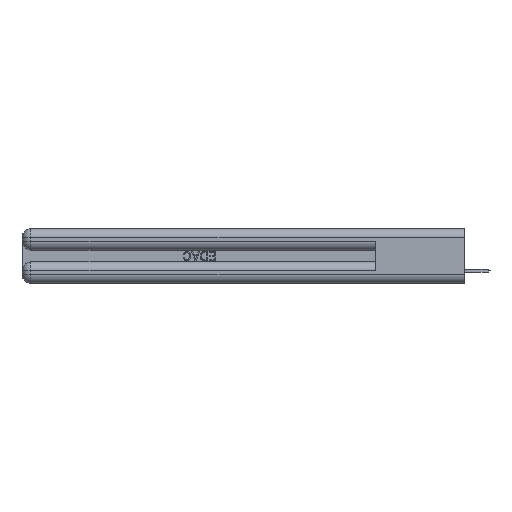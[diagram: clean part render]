
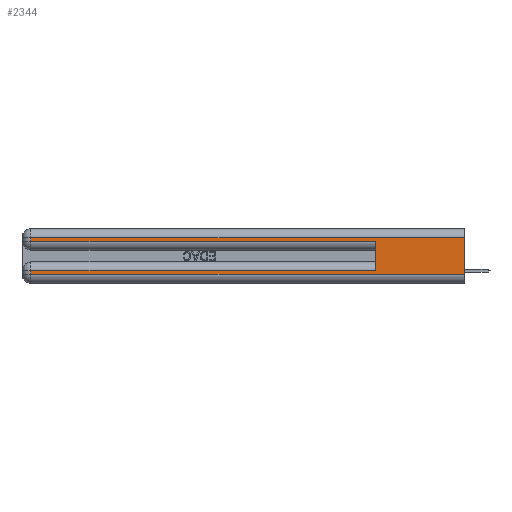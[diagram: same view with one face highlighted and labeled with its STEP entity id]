
A CAD part, left-side view. The second image highlights one B-rep face of the part: STEP entity #2344.
In plain terms, the highlighted planar face has unit normal (-1, 0, 0).
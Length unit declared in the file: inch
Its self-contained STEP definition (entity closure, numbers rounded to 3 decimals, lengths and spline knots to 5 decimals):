
#362 = VERTEX_POINT ( 'NONE', #38964 ) ;
#955 = EDGE_CURVE ( 'NONE', #15103, #29550, #20233, .T. ) ;
#1811 = CARTESIAN_POINT ( 'NONE',  ( 0., 2.94, 0.31 ) ) ;
#2344 = ADVANCED_FACE ( 'NONE', ( #28671 ), #14030, .F. ) ;
#2415 = ORIENTED_EDGE ( 'NONE', *, *, #22711, .F. ) ;
#2504 = LINE ( 'NONE', #26311, #26095 ) ;
#2969 = DIRECTION ( 'NONE',  ( 0., 0., -1. ) ) ;
#3115 = DIRECTION ( 'NONE',  ( 0., -1., 0. ) ) ;
#3134 = VERTEX_POINT ( 'NONE', #21106 ) ;
#3225 = EDGE_CURVE ( 'NONE', #16773, #38632, #2504, .T. ) ;
#3270 = DIRECTION ( 'NONE',  ( 0., 0., -1. ) ) ;
#4469 = CARTESIAN_POINT ( 'NONE',  ( 0., 2.94, 0.085 ) ) ;
#4632 = ORIENTED_EDGE ( 'NONE', *, *, #32119, .T. ) ;
#5028 = LINE ( 'NONE', #17285, #19050 ) ;
#5137 = DIRECTION ( 'NONE',  ( 0., 0., 1. ) ) ;
#5389 = DIRECTION ( 'NONE',  ( 0., 0., -1. ) ) ;
#7161 = VECTOR ( 'NONE', #3270, 39.37008 ) ;
#7966 = DIRECTION ( 'NONE',  ( 0., 1., 0. ) ) ;
#8090 = CARTESIAN_POINT ( 'NONE',  ( 0., 2.94, 0.06 ) ) ;
#8516 = DIRECTION ( 'NONE',  ( 0., 1., 0. ) ) ;
#8876 = CARTESIAN_POINT ( 'NONE',  ( 0., 0.6, 0.085 ) ) ;
#9044 = VERTEX_POINT ( 'NONE', #1811 ) ;
#10398 = EDGE_CURVE ( 'NONE', #43129, #38632, #41412, .T. ) ;
#12212 = EDGE_CURVE ( 'NONE', #29550, #43129, #5028, .T. ) ;
#14030 = PLANE ( 'NONE',  #15608 ) ;
#15103 = VERTEX_POINT ( 'NONE', #8876 ) ;
#15608 = AXIS2_PLACEMENT_3D ( 'NONE', #43233, #17788, #35631 ) ;
#16773 = VERTEX_POINT ( 'NONE', #19461 ) ;
#17285 = CARTESIAN_POINT ( 'NONE',  ( 0., 2.94, 0.37 ) ) ;
#17788 = DIRECTION ( 'NONE',  ( 1., 0., 0. ) ) ;
#19050 = VECTOR ( 'NONE', #2969, 39.37008 ) ;
#19461 = CARTESIAN_POINT ( 'NONE',  ( 0., 0., 0.31 ) ) ;
#20233 = LINE ( 'NONE', #29545, #36537 ) ;
#20673 = LINE ( 'NONE', #24368, #7161 ) ;
#21061 = CARTESIAN_POINT ( 'NONE',  ( 0., 0., 0.285 ) ) ;
#21106 = CARTESIAN_POINT ( 'NONE',  ( 0., 0.6, 0.285 ) ) ;
#21203 = VECTOR ( 'NONE', #8516, 39.37008 ) ;
#21588 = LINE ( 'NONE', #26998, #41427 ) ;
#22084 = VECTOR ( 'NONE', #33258, 39.37008 ) ;
#22711 = EDGE_CURVE ( 'NONE', #15103, #3134, #21588, .T. ) ;
#23289 = LINE ( 'NONE', #21061, #41484 ) ;
#23952 = ORIENTED_EDGE ( 'NONE', *, *, #37286, .T. ) ;
#23984 = LINE ( 'NONE', #33750, #21203 ) ;
#24368 = CARTESIAN_POINT ( 'NONE',  ( 0., 2.94, 0.37 ) ) ;
#25414 = ORIENTED_EDGE ( 'NONE', *, *, #955, .T. ) ;
#25744 = ORIENTED_EDGE ( 'NONE', *, *, #10398, .T. ) ;
#26095 = VECTOR ( 'NONE', #5389, 39.37008 ) ;
#26311 = CARTESIAN_POINT ( 'NONE',  ( 0., 0., 0.37 ) ) ;
#26807 = ORIENTED_EDGE ( 'NONE', *, *, #12212, .T. ) ;
#26998 = CARTESIAN_POINT ( 'NONE',  ( 0., 0.6, 0.145 ) ) ;
#28671 = FACE_OUTER_BOUND ( 'NONE', #34895, .T. ) ;
#29325 = CARTESIAN_POINT ( 'NONE',  ( 0., 0., 0.06 ) ) ;
#29545 = CARTESIAN_POINT ( 'NONE',  ( 0., 0., 0.085 ) ) ;
#29550 = VERTEX_POINT ( 'NONE', #4469 ) ;
#32119 = EDGE_CURVE ( 'NONE', #9044, #362, #20673, .T. ) ;
#32434 = EDGE_CURVE ( 'NONE', #16773, #9044, #23984, .T. ) ;
#33258 = DIRECTION ( 'NONE',  ( 0., -1., 0. ) ) ;
#33750 = CARTESIAN_POINT ( 'NONE',  ( 0., 0., 0.31 ) ) ;
#34895 = EDGE_LOOP ( 'NONE', ( #36725, #38766, #4632, #23952, #2415, #25414, #26807, #25744 ) ) ;
#35631 = DIRECTION ( 'NONE',  ( 0., 0., -1. ) ) ;
#36537 = VECTOR ( 'NONE', #7966, 39.37008 ) ;
#36725 = ORIENTED_EDGE ( 'NONE', *, *, #3225, .F. ) ;
#37286 = EDGE_CURVE ( 'NONE', #362, #3134, #23289, .T. ) ;
#38632 = VERTEX_POINT ( 'NONE', #40495 ) ;
#38766 = ORIENTED_EDGE ( 'NONE', *, *, #32434, .T. ) ;
#38964 = CARTESIAN_POINT ( 'NONE',  ( 0., 2.94, 0.285 ) ) ;
#40495 = CARTESIAN_POINT ( 'NONE',  ( 0., 0., 0.06 ) ) ;
#41412 = LINE ( 'NONE', #29325, #22084 ) ;
#41427 = VECTOR ( 'NONE', #5137, 39.37008 ) ;
#41484 = VECTOR ( 'NONE', #3115, 39.37008 ) ;
#43129 = VERTEX_POINT ( 'NONE', #8090 ) ;
#43233 = CARTESIAN_POINT ( 'NONE',  ( 0., 0., 0.37 ) ) ;
